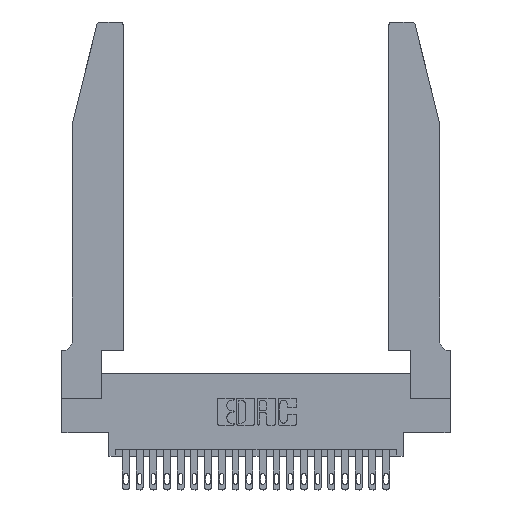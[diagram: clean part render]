
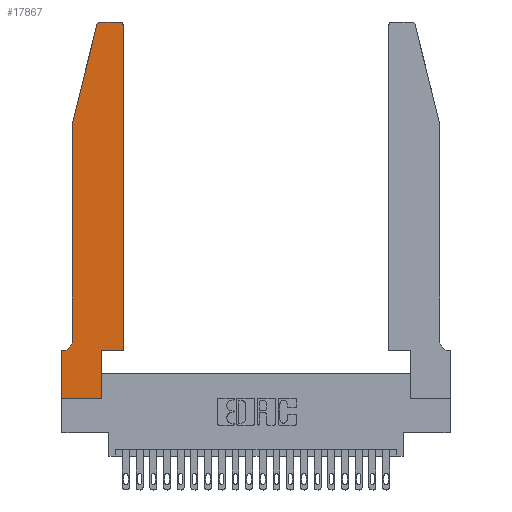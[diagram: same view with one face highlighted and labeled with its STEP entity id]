
A CAD part, top view. The second image highlights one B-rep face of the part: STEP entity #17867.
In plain terms, the highlighted planar face has unit normal (0, 0, 1).
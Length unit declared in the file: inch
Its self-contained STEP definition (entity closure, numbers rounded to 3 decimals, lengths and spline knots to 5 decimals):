
#355 = ORIENTED_EDGE ( 'NONE', *, *, #10840, .T. ) ;
#775 = EDGE_CURVE ( 'NONE', #1916, #4100, #9100, .T. ) ;
#806 = ORIENTED_EDGE ( 'NONE', *, *, #7363, .T. ) ;
#848 = EDGE_CURVE ( 'NONE', #23216, #1916, #7933, .T. ) ;
#1336 = CARTESIAN_POINT ( 'NONE',  ( 0.4505, 0.35, 0.37 ) ) ;
#1670 = LINE ( 'NONE', #5574, #13892 ) ;
#1860 = LINE ( 'NONE', #21646, #19454 ) ;
#1912 = DIRECTION ( 'NONE',  ( 1., 0., 0. ) ) ;
#1916 = VERTEX_POINT ( 'NONE', #19152 ) ;
#1983 = CARTESIAN_POINT ( 'NONE',  ( 0., 0., 0.37 ) ) ;
#2044 = CARTESIAN_POINT ( 'NONE',  ( 0.4505, 0.35, 0.37 ) ) ;
#2409 = EDGE_CURVE ( 'NONE', #16939, #15069, #1670, .T. ) ;
#2795 = DIRECTION ( 'NONE',  ( 0., 0., 1. ) ) ;
#3111 = CARTESIAN_POINT ( 'NONE',  ( 0.0755, 0.42, 0.37 ) ) ;
#3117 = CARTESIAN_POINT ( 'NONE',  ( 0.0755, 0.35, 0.37 ) ) ;
#3452 = ORIENTED_EDGE ( 'NONE', *, *, #6012, .T. ) ;
#3525 = DIRECTION ( 'NONE',  ( 1., 0., 0. ) ) ;
#3849 = DIRECTION ( 'NONE',  ( 0., 1., 0. ) ) ;
#4100 = VERTEX_POINT ( 'NONE', #5571 ) ;
#4396 = VERTEX_POINT ( 'NONE', #21383 ) ;
#4584 = PLANE ( 'NONE',  #23032 ) ;
#4795 = ORIENTED_EDGE ( 'NONE', *, *, #2409, .T. ) ;
#5115 = VECTOR ( 'NONE', #21295, 39.37008 ) ;
#5176 = CIRCLE ( 'NONE', #8599, 0.03 ) ;
#5316 = DIRECTION ( 'NONE',  ( 0., 1., 0. ) ) ;
#5466 = FACE_OUTER_BOUND ( 'NONE', #7094, .T. ) ;
#5571 = CARTESIAN_POINT ( 'NONE',  ( 0., 0.35, 0.37 ) ) ;
#5574 = CARTESIAN_POINT ( 'NONE',  ( 0.2605, 2.75, 0.37 ) ) ;
#5609 = CARTESIAN_POINT ( 'NONE',  ( 0.284, 2.75, 0.37 ) ) ;
#6012 = EDGE_CURVE ( 'NONE', #22406, #20404, #13638, .T. ) ;
#6220 = CARTESIAN_POINT ( 'NONE',  ( 0.0055, 0.42, 0.37 ) ) ;
#7094 = EDGE_LOOP ( 'NONE', ( #4795, #9344, #18419, #18902, #9009, #19432, #17219, #11336, #806, #3452, #355, #7187 ) ) ;
#7187 = ORIENTED_EDGE ( 'NONE', *, *, #13878, .T. ) ;
#7363 = EDGE_CURVE ( 'NONE', #4396, #22406, #9286, .T. ) ;
#7933 = CIRCLE ( 'NONE', #13233, 0.07 ) ;
#8025 = DIRECTION ( 'NONE',  ( -1., 0., 0. ) ) ;
#8385 = CARTESIAN_POINT ( 'NONE',  ( 0., 0.35, 0.37 ) ) ;
#8599 = AXIS2_PLACEMENT_3D ( 'NONE', #9949, #18968, #13740 ) ;
#9009 = ORIENTED_EDGE ( 'NONE', *, *, #848, .T. ) ;
#9100 = LINE ( 'NONE', #3117, #5115 ) ;
#9286 = LINE ( 'NONE', #16695, #9552 ) ;
#9344 = ORIENTED_EDGE ( 'NONE', *, *, #22012, .T. ) ;
#9552 = VECTOR ( 'NONE', #5316, 39.37008 ) ;
#9864 = DIRECTION ( 'NONE',  ( 0., 0., -1. ) ) ;
#9949 = CARTESIAN_POINT ( 'NONE',  ( 0.284, 2.72, 0.37 ) ) ;
#10742 = DIRECTION ( 'NONE',  ( 0., 0., 1. ) ) ;
#10840 = EDGE_CURVE ( 'NONE', #20404, #13707, #20313, .T. ) ;
#11336 = ORIENTED_EDGE ( 'NONE', *, *, #19908, .T. ) ;
#12085 = CARTESIAN_POINT ( 'NONE',  ( 0.4505, 2.72, 0.37 ) ) ;
#12179 = LINE ( 'NONE', #16131, #20708 ) ;
#12484 = DIRECTION ( 'NONE',  ( 0., -1., 0. ) ) ;
#12696 = CARTESIAN_POINT ( 'NONE',  ( 0.0755, 2., 0.37 ) ) ;
#13190 = VERTEX_POINT ( 'NONE', #12696 ) ;
#13233 = AXIS2_PLACEMENT_3D ( 'NONE', #6220, #9864, #8025 ) ;
#13378 = CARTESIAN_POINT ( 'NONE',  ( 0.25487, 2.72718, 0.37 ) ) ;
#13615 = DIRECTION ( 'NONE',  ( 1., 0., 0. ) ) ;
#13638 = LINE ( 'NONE', #18924, #22431 ) ;
#13707 = VERTEX_POINT ( 'NONE', #12085 ) ;
#13740 = DIRECTION ( 'NONE',  ( 1., 0., 0. ) ) ;
#13878 = EDGE_CURVE ( 'NONE', #13707, #16939, #17876, .T. ) ;
#13892 = VECTOR ( 'NONE', #14602, 39.37008 ) ;
#14587 = CARTESIAN_POINT ( 'NONE',  ( 0.0755, 2., 0.37 ) ) ;
#14602 = DIRECTION ( 'NONE',  ( -1., 0., 0. ) ) ;
#15069 = VERTEX_POINT ( 'NONE', #5609 ) ;
#15098 = VERTEX_POINT ( 'NONE', #1983 ) ;
#15770 = VECTOR ( 'NONE', #3849, 39.37008 ) ;
#15929 = VERTEX_POINT ( 'NONE', #13378 ) ;
#16131 = CARTESIAN_POINT ( 'NONE',  ( 0., 0., 0.37 ) ) ;
#16695 = CARTESIAN_POINT ( 'NONE',  ( 0.2865, 0.35, 0.37 ) ) ;
#16737 = CARTESIAN_POINT ( 'NONE',  ( 0.4205, 2.75, 0.37 ) ) ;
#16939 = VERTEX_POINT ( 'NONE', #16737 ) ;
#16968 = CARTESIAN_POINT ( 'NONE',  ( 0.2865, 0.35, 0.37 ) ) ;
#17219 = ORIENTED_EDGE ( 'NONE', *, *, #20481, .T. ) ;
#17648 = EDGE_CURVE ( 'NONE', #15929, #13190, #23386, .T. ) ;
#17736 = LINE ( 'NONE', #14587, #19433 ) ;
#17759 = DIRECTION ( 'NONE',  ( 0., -1., 0. ) ) ;
#17867 = ADVANCED_FACE ( 'NONE', ( #5466 ), #4584, .T. ) ;
#17876 = CIRCLE ( 'NONE', #19942, 0.03 ) ;
#18419 = ORIENTED_EDGE ( 'NONE', *, *, #17648, .T. ) ;
#18902 = ORIENTED_EDGE ( 'NONE', *, *, #21073, .T. ) ;
#18924 = CARTESIAN_POINT ( 'NONE',  ( 0.4505, 0.35, 0.37 ) ) ;
#18968 = DIRECTION ( 'NONE',  ( 0., 0., 1. ) ) ;
#19152 = CARTESIAN_POINT ( 'NONE',  ( 0.0055, 0.35, 0.37 ) ) ;
#19432 = ORIENTED_EDGE ( 'NONE', *, *, #775, .T. ) ;
#19433 = VECTOR ( 'NONE', #12484, 39.37008 ) ;
#19454 = VECTOR ( 'NONE', #17759, 39.37008 ) ;
#19813 = CARTESIAN_POINT ( 'NONE',  ( 0.4205, 2.72, 0.37 ) ) ;
#19908 = EDGE_CURVE ( 'NONE', #15098, #4396, #12179, .T. ) ;
#19942 = AXIS2_PLACEMENT_3D ( 'NONE', #19813, #10742, #3525 ) ;
#20313 = LINE ( 'NONE', #2044, #15770 ) ;
#20404 = VERTEX_POINT ( 'NONE', #1336 ) ;
#20481 = EDGE_CURVE ( 'NONE', #4100, #15098, #1860, .T. ) ;
#20552 = VECTOR ( 'NONE', #22557, 39.37008 ) ;
#20708 = VECTOR ( 'NONE', #1912, 39.37008 ) ;
#21073 = EDGE_CURVE ( 'NONE', #13190, #23216, #17736, .T. ) ;
#21295 = DIRECTION ( 'NONE',  ( -1., 0., 0. ) ) ;
#21383 = CARTESIAN_POINT ( 'NONE',  ( 0.2865, 0., 0.37 ) ) ;
#21646 = CARTESIAN_POINT ( 'NONE',  ( 0., 0., 0.37 ) ) ;
#22012 = EDGE_CURVE ( 'NONE', #15069, #15929, #5176, .T. ) ;
#22331 = CARTESIAN_POINT ( 'NONE',  ( 0.0755, 2., 0.37 ) ) ;
#22406 = VERTEX_POINT ( 'NONE', #16968 ) ;
#22431 = VECTOR ( 'NONE', #22488, 39.37008 ) ;
#22488 = DIRECTION ( 'NONE',  ( 1., 0., 0. ) ) ;
#22557 = DIRECTION ( 'NONE',  ( -0.239, -0.971, 0. ) ) ;
#23032 = AXIS2_PLACEMENT_3D ( 'NONE', #8385, #2795, #13615 ) ;
#23216 = VERTEX_POINT ( 'NONE', #3111 ) ;
#23386 = LINE ( 'NONE', #22331, #20552 ) ;
